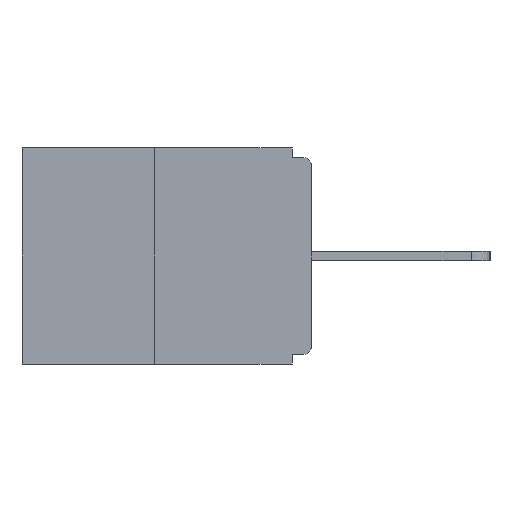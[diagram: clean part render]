
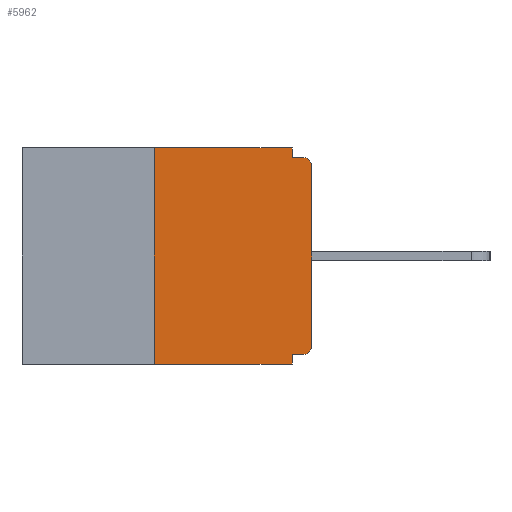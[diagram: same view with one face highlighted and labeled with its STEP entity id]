
A CAD part, left-side view. The second image highlights one B-rep face of the part: STEP entity #5962.
In plain terms, the highlighted planar face has unit normal (-1, 0, 0).
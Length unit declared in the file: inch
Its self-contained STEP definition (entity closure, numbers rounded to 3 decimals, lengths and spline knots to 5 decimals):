
#259 = CARTESIAN_POINT ( 'NONE',  ( 0., 0., -0.328 ) ) ;
#282 = CARTESIAN_POINT ( 'NONE',  ( 0., 0., -0.015 ) ) ;
#370 = CARTESIAN_POINT ( 'NONE',  ( 0., 0.031, -0.343 ) ) ;
#415 = EDGE_CURVE ( 'NONE', #6561, #12277, #6079, .T. ) ;
#842 = DIRECTION ( 'NONE',  ( 0., 0., -1. ) ) ;
#874 = VERTEX_POINT ( 'NONE', #2289 ) ;
#934 = CARTESIAN_POINT ( 'NONE',  ( 0., 0.031, 0. ) ) ;
#1258 = EDGE_CURVE ( 'NONE', #10561, #5006, #7868, .T. ) ;
#1282 = VERTEX_POINT ( 'NONE', #1715 ) ;
#1555 = DIRECTION ( 'NONE',  ( 0., 0., 1. ) ) ;
#1672 = CIRCLE ( 'NONE', #10845, 0.015 ) ;
#1715 = CARTESIAN_POINT ( 'NONE',  ( 0., 0., -0.313 ) ) ;
#2030 = EDGE_LOOP ( 'NONE', ( #6259, #6611, #5286, #5099, #2725, #3801, #5864, #4103, #2295, #11981 ) ) ;
#2144 = VECTOR ( 'NONE', #1555, 39.37008 ) ;
#2194 = DIRECTION ( 'NONE',  ( 0., 0., -1. ) ) ;
#2289 = CARTESIAN_POINT ( 'NONE',  ( 0., 0.015, -0.328 ) ) ;
#2295 = ORIENTED_EDGE ( 'NONE', *, *, #2296, .F. ) ;
#2296 = EDGE_CURVE ( 'NONE', #12326, #10128, #12551, .T. ) ;
#2454 = DIRECTION ( 'NONE',  ( 0., 0., -1. ) ) ;
#2464 = FACE_OUTER_BOUND ( 'NONE', #2030, .T. ) ;
#2552 = VECTOR ( 'NONE', #3277, 39.37008 ) ;
#2725 = ORIENTED_EDGE ( 'NONE', *, *, #12137, .F. ) ;
#2811 = EDGE_CURVE ( 'NONE', #5006, #12326, #6838, .T. ) ;
#2866 = CIRCLE ( 'NONE', #10116, 0.015 ) ;
#3277 = DIRECTION ( 'NONE',  ( 0., 1., 0. ) ) ;
#3801 = ORIENTED_EDGE ( 'NONE', *, *, #9244, .T. ) ;
#4103 = ORIENTED_EDGE ( 'NONE', *, *, #11076, .T. ) ;
#4220 = VECTOR ( 'NONE', #7067, 39.37008 ) ;
#4225 = LINE ( 'NONE', #259, #2552 ) ;
#4418 = VERTEX_POINT ( 'NONE', #12004 ) ;
#4598 = CARTESIAN_POINT ( 'NONE',  ( 0., 0., 0. ) ) ;
#4726 = CARTESIAN_POINT ( 'NONE',  ( 0., 0.015, -0.03 ) ) ;
#5006 = VERTEX_POINT ( 'NONE', #934 ) ;
#5099 = ORIENTED_EDGE ( 'NONE', *, *, #8932, .F. ) ;
#5127 = DIRECTION ( 'NONE',  ( 0., -1., 0. ) ) ;
#5211 = DIRECTION ( 'NONE',  ( 1., 0., 0. ) ) ;
#5266 = CARTESIAN_POINT ( 'NONE',  ( 0., 0.46, -0.343 ) ) ;
#5286 = ORIENTED_EDGE ( 'NONE', *, *, #415, .T. ) ;
#5458 = LINE ( 'NONE', #370, #7575 ) ;
#5551 = CARTESIAN_POINT ( 'NONE',  ( 0., 0.031, -0.343 ) ) ;
#5741 = DIRECTION ( 'NONE',  ( 0., 0., 1. ) ) ;
#5864 = ORIENTED_EDGE ( 'NONE', *, *, #7306, .T. ) ;
#5870 = LINE ( 'NONE', #4598, #7624 ) ;
#5962 = ADVANCED_FACE ( 'NONE', ( #2464 ), #7296, .F. ) ;
#6079 = LINE ( 'NONE', #5266, #10746 ) ;
#6259 = ORIENTED_EDGE ( 'NONE', *, *, #1258, .F. ) ;
#6453 = DIRECTION ( 'NONE',  ( -1., 0., 0. ) ) ;
#6561 = VERTEX_POINT ( 'NONE', #12406 ) ;
#6611 = ORIENTED_EDGE ( 'NONE', *, *, #10208, .F. ) ;
#6838 = LINE ( 'NONE', #13207, #7124 ) ;
#6853 = CARTESIAN_POINT ( 'NONE',  ( 0., 0.25, 0. ) ) ;
#6859 = CARTESIAN_POINT ( 'NONE',  ( 0., 0.46, 0. ) ) ;
#7067 = DIRECTION ( 'NONE',  ( 0., -1., 0. ) ) ;
#7081 = DIRECTION ( 'NONE',  ( 0., -1., 0. ) ) ;
#7124 = VECTOR ( 'NONE', #9967, 39.37008 ) ;
#7296 = PLANE ( 'NONE',  #13154 ) ;
#7306 = EDGE_CURVE ( 'NONE', #1282, #4418, #5870, .T. ) ;
#7397 = CARTESIAN_POINT ( 'NONE',  ( 0., 0.015, -0.313 ) ) ;
#7471 = DIRECTION ( 'NONE',  ( 0., 0., -1. ) ) ;
#7575 = VECTOR ( 'NONE', #2454, 39.37008 ) ;
#7624 = VECTOR ( 'NONE', #5741, 39.37008 ) ;
#7868 = LINE ( 'NONE', #6859, #4220 ) ;
#8337 = CARTESIAN_POINT ( 'NONE',  ( 0., 0.031, -0.328 ) ) ;
#8932 = EDGE_CURVE ( 'NONE', #11216, #12277, #5458, .T. ) ;
#9244 = EDGE_CURVE ( 'NONE', #874, #1282, #2866, .T. ) ;
#9967 = DIRECTION ( 'NONE',  ( 0., 0., -1. ) ) ;
#10116 = AXIS2_PLACEMENT_3D ( 'NONE', #7397, #6453, #7471 ) ;
#10128 = VERTEX_POINT ( 'NONE', #11598 ) ;
#10208 = EDGE_CURVE ( 'NONE', #6561, #10561, #12953, .T. ) ;
#10561 = VERTEX_POINT ( 'NONE', #12658 ) ;
#10605 = CARTESIAN_POINT ( 'NONE',  ( 0., 0.46, 0. ) ) ;
#10746 = VECTOR ( 'NONE', #7081, 39.37008 ) ;
#10845 = AXIS2_PLACEMENT_3D ( 'NONE', #4726, #12031, #842 ) ;
#11076 = EDGE_CURVE ( 'NONE', #4418, #10128, #1672, .T. ) ;
#11216 = VERTEX_POINT ( 'NONE', #8337 ) ;
#11259 = VECTOR ( 'NONE', #5127, 39.37008 ) ;
#11598 = CARTESIAN_POINT ( 'NONE',  ( 0., 0.015, -0.015 ) ) ;
#11704 = CARTESIAN_POINT ( 'NONE',  ( 0., 0.031, -0.015 ) ) ;
#11981 = ORIENTED_EDGE ( 'NONE', *, *, #2811, .F. ) ;
#12004 = CARTESIAN_POINT ( 'NONE',  ( 0., 0., -0.03 ) ) ;
#12031 = DIRECTION ( 'NONE',  ( -1., 0., 0. ) ) ;
#12137 = EDGE_CURVE ( 'NONE', #874, #11216, #4225, .T. ) ;
#12277 = VERTEX_POINT ( 'NONE', #5551 ) ;
#12326 = VERTEX_POINT ( 'NONE', #11704 ) ;
#12406 = CARTESIAN_POINT ( 'NONE',  ( 0., 0.25, -0.343 ) ) ;
#12551 = LINE ( 'NONE', #282, #11259 ) ;
#12658 = CARTESIAN_POINT ( 'NONE',  ( 0., 0.25, 0. ) ) ;
#12953 = LINE ( 'NONE', #6853, #2144 ) ;
#13154 = AXIS2_PLACEMENT_3D ( 'NONE', #10605, #5211, #2194 ) ;
#13207 = CARTESIAN_POINT ( 'NONE',  ( 0., 0.031, 0. ) ) ;
